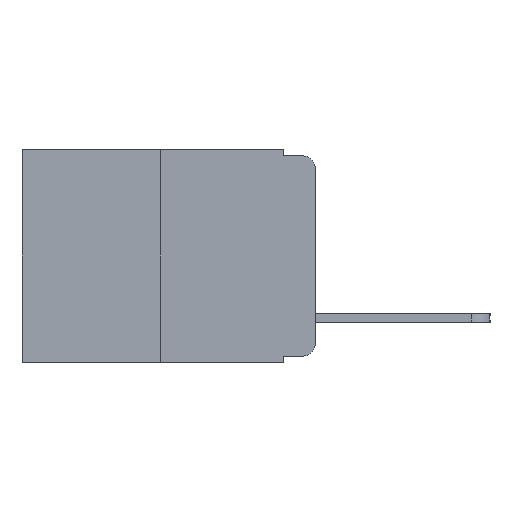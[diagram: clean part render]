
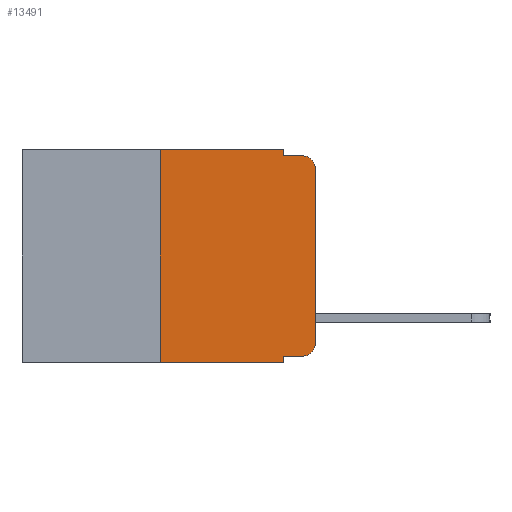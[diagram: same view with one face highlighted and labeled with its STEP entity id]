
A CAD part, left-side view. The second image highlights one B-rep face of the part: STEP entity #13491.
In plain terms, the highlighted planar face has unit normal (-1, 0, 0).
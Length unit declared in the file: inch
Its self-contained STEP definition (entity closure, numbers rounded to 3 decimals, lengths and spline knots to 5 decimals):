
#367 = AXIS2_PLACEMENT_3D ( 'NONE', #4171, #11626, #5293 ) ;
#442 = DIRECTION ( 'NONE',  ( 0., -1., 0. ) ) ;
#454 = ORIENTED_EDGE ( 'NONE', *, *, #1228, .F. ) ;
#505 = CARTESIAN_POINT ( 'NONE',  ( 0., 0.051, -0.01 ) ) ;
#622 = CARTESIAN_POINT ( 'NONE',  ( 0., 0.051, 0. ) ) ;
#867 = VECTOR ( 'NONE', #13218, 39.37008 ) ;
#948 = ORIENTED_EDGE ( 'NONE', *, *, #9812, .F. ) ;
#1228 = EDGE_CURVE ( 'NONE', #12037, #12778, #2610, .T. ) ;
#1259 = ORIENTED_EDGE ( 'NONE', *, *, #1908, .T. ) ;
#1322 = CARTESIAN_POINT ( 'NONE',  ( 0., 0.02, -0.03 ) ) ;
#1336 = VERTEX_POINT ( 'NONE', #3669 ) ;
#1721 = DIRECTION ( 'NONE',  ( 0., 0., -1. ) ) ;
#1722 = EDGE_CURVE ( 'NONE', #2819, #9301, #2254, .T. ) ;
#1767 = DIRECTION ( 'NONE',  ( -1., 0., 0. ) ) ;
#1908 = EDGE_CURVE ( 'NONE', #7437, #1336, #8883, .T. ) ;
#2203 = CARTESIAN_POINT ( 'NONE',  ( 0., 0.051, -0.333 ) ) ;
#2254 = LINE ( 'NONE', #505, #5435 ) ;
#2319 = EDGE_LOOP ( 'NONE', ( #1259, #5461, #9942, #948, #10919, #454, #11277, #7504, #9796, #6842 ) ) ;
#2402 = DIRECTION ( 'NONE',  ( 0., 0., -1. ) ) ;
#2503 = CARTESIAN_POINT ( 'NONE',  ( 0., 0.473, 0. ) ) ;
#2610 = LINE ( 'NONE', #5559, #13543 ) ;
#2819 = VERTEX_POINT ( 'NONE', #7734 ) ;
#3204 = VECTOR ( 'NONE', #10423, 39.37008 ) ;
#3669 = CARTESIAN_POINT ( 'NONE',  ( 0., 0., -0.03 ) ) ;
#4171 = CARTESIAN_POINT ( 'NONE',  ( 0., 0.473, 0. ) ) ;
#4755 = DIRECTION ( 'NONE',  ( 0., -1., 0. ) ) ;
#4817 = LINE ( 'NONE', #2503, #10446 ) ;
#4832 = LINE ( 'NONE', #7205, #10463 ) ;
#5123 = AXIS2_PLACEMENT_3D ( 'NONE', #1322, #8813, #2402 ) ;
#5293 = DIRECTION ( 'NONE',  ( 0., 0., -1. ) ) ;
#5378 = EDGE_CURVE ( 'NONE', #12778, #9348, #4817, .T. ) ;
#5410 = EDGE_CURVE ( 'NONE', #12037, #5619, #9463, .T. ) ;
#5435 = VECTOR ( 'NONE', #442, 39.37008 ) ;
#5461 = ORIENTED_EDGE ( 'NONE', *, *, #7909, .T. ) ;
#5559 = CARTESIAN_POINT ( 'NONE',  ( 0., 0.25, 0. ) ) ;
#5619 = VERTEX_POINT ( 'NONE', #13483 ) ;
#6640 = VECTOR ( 'NONE', #4755, 39.37008 ) ;
#6842 = ORIENTED_EDGE ( 'NONE', *, *, #10279, .T. ) ;
#6907 = FACE_OUTER_BOUND ( 'NONE', #2319, .T. ) ;
#6926 = CARTESIAN_POINT ( 'NONE',  ( 0., 0.051, 0. ) ) ;
#7031 = VERTEX_POINT ( 'NONE', #2203 ) ;
#7205 = CARTESIAN_POINT ( 'NONE',  ( 0., 0.051, -0.333 ) ) ;
#7437 = VERTEX_POINT ( 'NONE', #8062 ) ;
#7504 = ORIENTED_EDGE ( 'NONE', *, *, #11498, .F. ) ;
#7538 = EDGE_CURVE ( 'NONE', #7031, #11582, #4832, .T. ) ;
#7734 = CARTESIAN_POINT ( 'NONE',  ( 0., 0.051, -0.01 ) ) ;
#7909 = EDGE_CURVE ( 'NONE', #1336, #9301, #8666, .T. ) ;
#7963 = VECTOR ( 'NONE', #1721, 39.37008 ) ;
#8062 = CARTESIAN_POINT ( 'NONE',  ( 0., 0., -0.313 ) ) ;
#8150 = CARTESIAN_POINT ( 'NONE',  ( 0., 0.02, -0.333 ) ) ;
#8189 = CARTESIAN_POINT ( 'NONE',  ( 0., 0.02, -0.313 ) ) ;
#8264 = CARTESIAN_POINT ( 'NONE',  ( 0., 0.25, 0. ) ) ;
#8666 = CIRCLE ( 'NONE', #5123, 0.02 ) ;
#8813 = DIRECTION ( 'NONE',  ( -1., 0., 0. ) ) ;
#8883 = LINE ( 'NONE', #11308, #3204 ) ;
#9053 = LINE ( 'NONE', #6926, #867 ) ;
#9225 = DIRECTION ( 'NONE',  ( 0., 0., -1. ) ) ;
#9301 = VERTEX_POINT ( 'NONE', #11424 ) ;
#9348 = VERTEX_POINT ( 'NONE', #12587 ) ;
#9463 = LINE ( 'NONE', #11087, #6640 ) ;
#9796 = ORIENTED_EDGE ( 'NONE', *, *, #7538, .T. ) ;
#9812 = EDGE_CURVE ( 'NONE', #9348, #2819, #10726, .T. ) ;
#9942 = ORIENTED_EDGE ( 'NONE', *, *, #1722, .F. ) ;
#10279 = EDGE_CURVE ( 'NONE', #11582, #7437, #13677, .T. ) ;
#10423 = DIRECTION ( 'NONE',  ( 0., 0., 1. ) ) ;
#10446 = VECTOR ( 'NONE', #10999, 39.37008 ) ;
#10463 = VECTOR ( 'NONE', #13486, 39.37008 ) ;
#10561 = PLANE ( 'NONE',  #367 ) ;
#10726 = LINE ( 'NONE', #622, #7963 ) ;
#10919 = ORIENTED_EDGE ( 'NONE', *, *, #5378, .F. ) ;
#10999 = DIRECTION ( 'NONE',  ( 0., -1., 0. ) ) ;
#11087 = CARTESIAN_POINT ( 'NONE',  ( 0., 0.473, -0.343 ) ) ;
#11277 = ORIENTED_EDGE ( 'NONE', *, *, #5410, .T. ) ;
#11308 = CARTESIAN_POINT ( 'NONE',  ( 0., 0., 0. ) ) ;
#11424 = CARTESIAN_POINT ( 'NONE',  ( 0., 0.02, -0.01 ) ) ;
#11498 = EDGE_CURVE ( 'NONE', #7031, #5619, #9053, .T. ) ;
#11582 = VERTEX_POINT ( 'NONE', #8150 ) ;
#11626 = DIRECTION ( 'NONE',  ( 1., 0., 0. ) ) ;
#11682 = DIRECTION ( 'NONE',  ( 0., 0., 1. ) ) ;
#12037 = VERTEX_POINT ( 'NONE', #12200 ) ;
#12200 = CARTESIAN_POINT ( 'NONE',  ( 0., 0.25, -0.343 ) ) ;
#12587 = CARTESIAN_POINT ( 'NONE',  ( 0., 0.051, 0. ) ) ;
#12778 = VERTEX_POINT ( 'NONE', #8264 ) ;
#13218 = DIRECTION ( 'NONE',  ( 0., 0., -1. ) ) ;
#13483 = CARTESIAN_POINT ( 'NONE',  ( 0., 0.051, -0.343 ) ) ;
#13486 = DIRECTION ( 'NONE',  ( 0., -1., 0. ) ) ;
#13491 = ADVANCED_FACE ( 'NONE', ( #6907 ), #10561, .F. ) ;
#13543 = VECTOR ( 'NONE', #11682, 39.37008 ) ;
#13640 = AXIS2_PLACEMENT_3D ( 'NONE', #8189, #1767, #9225 ) ;
#13677 = CIRCLE ( 'NONE', #13640, 0.02 ) ;
